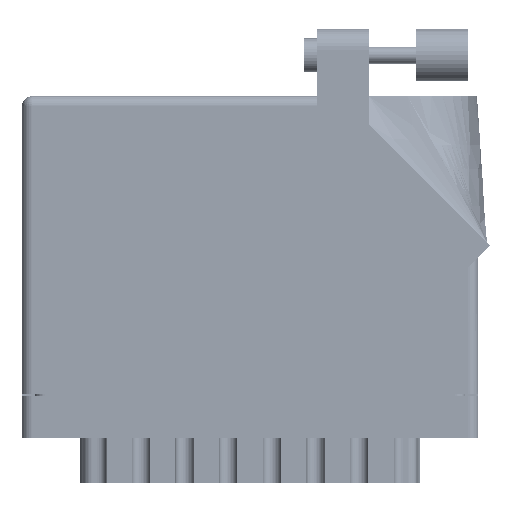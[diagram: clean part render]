
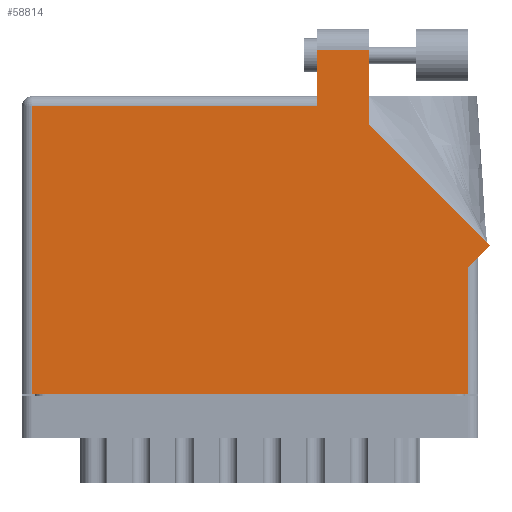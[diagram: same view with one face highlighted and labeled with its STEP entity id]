
A CAD part, front view. The second image highlights one B-rep face of the part: STEP entity #58814.
In plain terms, the highlighted face is planar.
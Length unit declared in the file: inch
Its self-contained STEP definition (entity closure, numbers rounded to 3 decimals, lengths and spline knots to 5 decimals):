
#708 = VERTEX_POINT ( 'NONE', #3151 ) ;
#817 = VECTOR ( 'NONE', #17201, 39.37008 ) ;
#1081 = VERTEX_POINT ( 'NONE', #67709 ) ;
#2529 = DIRECTION ( 'NONE',  ( -1., 0., 0. ) ) ;
#2652 = LINE ( 'NONE', #9149, #31204 ) ;
#3151 = CARTESIAN_POINT ( 'NONE',  ( 2.065, 2.05, 0. ) ) ;
#5328 = LINE ( 'NONE', #43567, #43194 ) ;
#5686 = ORIENTED_EDGE ( 'NONE', *, *, #54178, .T. ) ;
#5926 = VECTOR ( 'NONE', #53577, 39.37008 ) ;
#5986 = CARTESIAN_POINT ( 'NONE',  ( 2.065, 1.60942, 0. ) ) ;
#7200 = VECTOR ( 'NONE', #19828, 39.37008 ) ;
#7563 = VECTOR ( 'NONE', #7583, 39.37008 ) ;
#7583 = DIRECTION ( 'NONE',  ( -0.707, 0.707, 0. ) ) ;
#8718 = CARTESIAN_POINT ( 'NONE',  ( 0., 1.775, 0. ) ) ;
#9149 = CARTESIAN_POINT ( 'NONE',  ( 2.656, 0.815, 0. ) ) ;
#10476 = CARTESIAN_POINT ( 'NONE',  ( 0.062, 0., 0. ) ) ;
#10989 = CARTESIAN_POINT ( 'NONE',  ( 0., 1.713, 0. ) ) ;
#11217 = VECTOR ( 'NONE', #37940, 39.37008 ) ;
#11238 = ORIENTED_EDGE ( 'NONE', *, *, #25626, .T. ) ;
#16075 = ORIENTED_EDGE ( 'NONE', *, *, #62794, .T. ) ;
#17201 = DIRECTION ( 'NONE',  ( 0., 1., 0. ) ) ;
#18258 = AXIS2_PLACEMENT_3D ( 'NONE', #8718, #61524, #2529 ) ;
#18508 = VERTEX_POINT ( 'NONE', #36703 ) ;
#19828 = DIRECTION ( 'NONE',  ( -1., 0., 0. ) ) ;
#20940 = CARTESIAN_POINT ( 'NONE',  ( 1.758, 1.713, 0. ) ) ;
#22007 = VECTOR ( 'NONE', #40474, 39.37008 ) ;
#22884 = LINE ( 'NONE', #10476, #22007 ) ;
#25365 = CARTESIAN_POINT ( 'NONE',  ( 2.78871, 0.88571, 0. ) ) ;
#25626 = EDGE_CURVE ( 'NONE', #18508, #1081, #22884, .T. ) ;
#25736 = CARTESIAN_POINT ( 'NONE',  ( 2.718, 0.815, 0. ) ) ;
#26708 = DIRECTION ( 'NONE',  ( 0., 1., 0. ) ) ;
#28860 = ORIENTED_EDGE ( 'NONE', *, *, #57010, .T. ) ;
#31204 = VECTOR ( 'NONE', #26708, 39.37008 ) ;
#31587 = CARTESIAN_POINT ( 'NONE',  ( 2.656, 0., 0. ) ) ;
#32726 = ORIENTED_EDGE ( 'NONE', *, *, #48580, .T. ) ;
#33530 = ORIENTED_EDGE ( 'NONE', *, *, #39176, .T. ) ;
#35337 = CARTESIAN_POINT ( 'NONE',  ( 2.065, 1.60942, 0. ) ) ;
#36703 = CARTESIAN_POINT ( 'NONE',  ( 0.062, 1.713, 0. ) ) ;
#37940 = DIRECTION ( 'NONE',  ( 0.707, 0.707, 0. ) ) ;
#39176 = EDGE_CURVE ( 'NONE', #708, #71471, #46977, .T. ) ;
#39984 = LINE ( 'NONE', #25736, #11217 ) ;
#40474 = DIRECTION ( 'NONE',  ( 0., -1., 0. ) ) ;
#41736 = ORIENTED_EDGE ( 'NONE', *, *, #53209, .T. ) ;
#41942 = LINE ( 'NONE', #52084, #5926 ) ;
#43194 = VECTOR ( 'NONE', #49519, 39.37008 ) ;
#43567 = CARTESIAN_POINT ( 'NONE',  ( 1.758, 1.775, 0. ) ) ;
#43891 = PLANE ( 'NONE',  #18258 ) ;
#46977 = LINE ( 'NONE', #65316, #7200 ) ;
#48379 = CARTESIAN_POINT ( 'NONE',  ( 2.656, 0.753, 0. ) ) ;
#48580 = EDGE_CURVE ( 'NONE', #67851, #50915, #69578, .T. ) ;
#49519 = DIRECTION ( 'NONE',  ( 0., -1., 0. ) ) ;
#50795 = LINE ( 'NONE', #35337, #817 ) ;
#50915 = VERTEX_POINT ( 'NONE', #5986 ) ;
#51286 = CARTESIAN_POINT ( 'NONE',  ( 1.758, 2.05, 0. ) ) ;
#52084 = CARTESIAN_POINT ( 'NONE',  ( 0., 0., 0. ) ) ;
#52453 = DIRECTION ( 'NONE',  ( -1., 0., 0. ) ) ;
#53209 = EDGE_CURVE ( 'NONE', #50915, #708, #50795, .T. ) ;
#53577 = DIRECTION ( 'NONE',  ( 1., 0., 0. ) ) ;
#54178 = EDGE_CURVE ( 'NONE', #71471, #69429, #5328, .T. ) ;
#57010 = EDGE_CURVE ( 'NONE', #1081, #69355, #41942, .T. ) ;
#58570 = LINE ( 'NONE', #10989, #70529 ) ;
#58698 = ORIENTED_EDGE ( 'NONE', *, *, #75186, .T. ) ;
#58814 = ADVANCED_FACE ( 'NONE', ( #66165 ), #43891, .F. ) ;
#61524 = DIRECTION ( 'NONE',  ( 0., 0., -1. ) ) ;
#62794 = EDGE_CURVE ( 'NONE', #69355, #63624, #2652, .T. ) ;
#63624 = VERTEX_POINT ( 'NONE', #48379 ) ;
#64268 = CARTESIAN_POINT ( 'NONE',  ( 2.78871, 0.88571, 0. ) ) ;
#65316 = CARTESIAN_POINT ( 'NONE',  ( 1.758, 2.05, 0. ) ) ;
#66165 = FACE_OUTER_BOUND ( 'NONE', #74991, .T. ) ;
#67176 = EDGE_CURVE ( 'NONE', #69429, #18508, #58570, .T. ) ;
#67709 = CARTESIAN_POINT ( 'NONE',  ( 0.062, 0., 0. ) ) ;
#67851 = VERTEX_POINT ( 'NONE', #64268 ) ;
#69355 = VERTEX_POINT ( 'NONE', #31587 ) ;
#69429 = VERTEX_POINT ( 'NONE', #20940 ) ;
#69578 = LINE ( 'NONE', #25365, #7563 ) ;
#70529 = VECTOR ( 'NONE', #52453, 39.37008 ) ;
#71471 = VERTEX_POINT ( 'NONE', #51286 ) ;
#74991 = EDGE_LOOP ( 'NONE', ( #41736, #33530, #5686, #75443, #11238, #28860, #16075, #58698, #32726 ) ) ;
#75186 = EDGE_CURVE ( 'NONE', #63624, #67851, #39984, .T. ) ;
#75443 = ORIENTED_EDGE ( 'NONE', *, *, #67176, .T. ) ;
